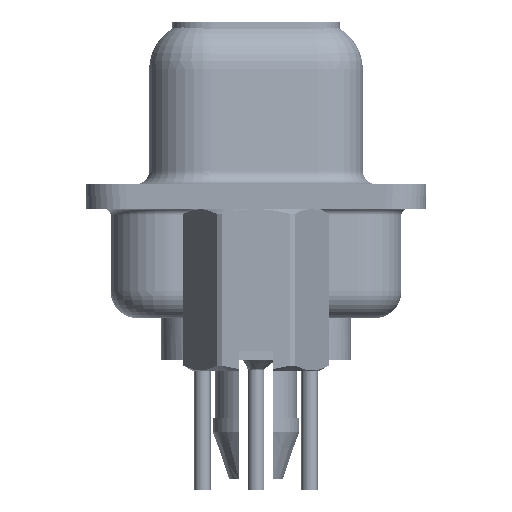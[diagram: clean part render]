
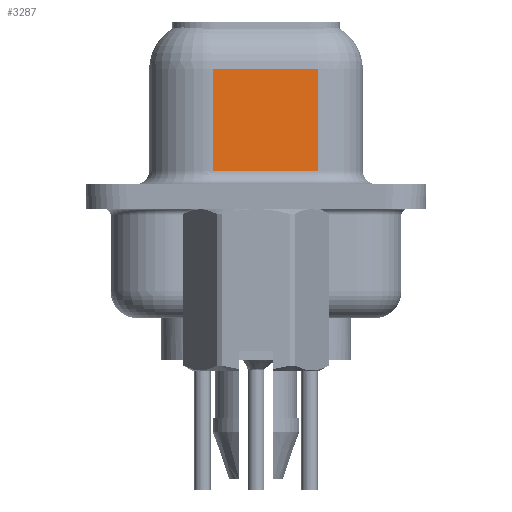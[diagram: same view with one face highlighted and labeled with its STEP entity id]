
A CAD part, left-side view. The second image highlights one B-rep face of the part: STEP entity #3287.
In plain terms, the highlighted planar face has unit normal (-0.985, -0.174, 0).
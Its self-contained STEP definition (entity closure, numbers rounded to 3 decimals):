
#232 = AXIS2_PLACEMENT_3D ( 'NONE', #35397, #7101, #22913 ) ;
#267 = VERTEX_POINT ( 'NONE', #33788 ) ;
#1306 = FACE_OUTER_BOUND ( 'NONE', #41039, .T. ) ;
#1421 = DIRECTION ( 'NONE',  ( -0.174, 0.985, 0. ) ) ;
#2619 = VECTOR ( 'NONE', #6544, 1000. ) ;
#3287 = ADVANCED_FACE ( 'NONE', ( #1306 ), #32684, .F. ) ;
#3516 = ORIENTED_EDGE ( 'NONE', *, *, #11378, .T. ) ;
#3948 = ORIENTED_EDGE ( 'NONE', *, *, #12875, .T. ) ;
#5441 = LINE ( 'NONE', #33529, #28103 ) ;
#6544 = DIRECTION ( 'NONE',  ( 0., 0., -1. ) ) ;
#7101 = DIRECTION ( 'NONE',  ( 0.985, 0.174, 0. ) ) ;
#7754 = VERTEX_POINT ( 'NONE', #35123 ) ;
#9224 = VERTEX_POINT ( 'NONE', #28017 ) ;
#10574 = EDGE_CURVE ( 'NONE', #267, #7754, #30292, .T. ) ;
#11378 = EDGE_CURVE ( 'NONE', #7754, #9224, #5441, .T. ) ;
#12875 = EDGE_CURVE ( 'NONE', #25032, #267, #17187, .T. ) ;
#17187 = LINE ( 'NONE', #29859, #24113 ) ;
#18796 = CARTESIAN_POINT ( 'NONE',  ( 5.038, -2.297, 4.7 ) ) ;
#19022 = ORIENTED_EDGE ( 'NONE', *, *, #27916, .F. ) ;
#21932 = LINE ( 'NONE', #25051, #2619 ) ;
#22913 = DIRECTION ( 'NONE',  ( -0.174, 0.985, 0. ) ) ;
#24113 = VECTOR ( 'NONE', #1421, 1000. ) ;
#24364 = DIRECTION ( 'NONE',  ( 0.174, -0.985, 0. ) ) ;
#25032 = VERTEX_POINT ( 'NONE', #18796 ) ;
#25051 = CARTESIAN_POINT ( 'NONE',  ( 5.038, -2.297, 6.45 ) ) ;
#27916 = EDGE_CURVE ( 'NONE', #25032, #9224, #21932, .T. ) ;
#28017 = CARTESIAN_POINT ( 'NONE',  ( 5.038, -2.297, 0.95 ) ) ;
#28103 = VECTOR ( 'NONE', #24364, 1000. ) ;
#29859 = CARTESIAN_POINT ( 'NONE',  ( 5.038, -2.297, 4.7 ) ) ;
#30045 = VECTOR ( 'NONE', #30908, 1000. ) ;
#30292 = LINE ( 'NONE', #40719, #30045 ) ;
#30908 = DIRECTION ( 'NONE',  ( 0., 0., -1. ) ) ;
#32684 = PLANE ( 'NONE',  #232 ) ;
#32762 = ORIENTED_EDGE ( 'NONE', *, *, #10574, .T. ) ;
#33529 = CARTESIAN_POINT ( 'NONE',  ( 5.038, -2.297, 0.95 ) ) ;
#33788 = CARTESIAN_POINT ( 'NONE',  ( 4.35, 1.603, 4.7 ) ) ;
#35123 = CARTESIAN_POINT ( 'NONE',  ( 4.35, 1.603, 0.95 ) ) ;
#35397 = CARTESIAN_POINT ( 'NONE',  ( 5.038, -2.297, 6.45 ) ) ;
#40719 = CARTESIAN_POINT ( 'NONE',  ( 4.35, 1.603, 6.45 ) ) ;
#41039 = EDGE_LOOP ( 'NONE', ( #19022, #3948, #32762, #3516 ) ) ;
